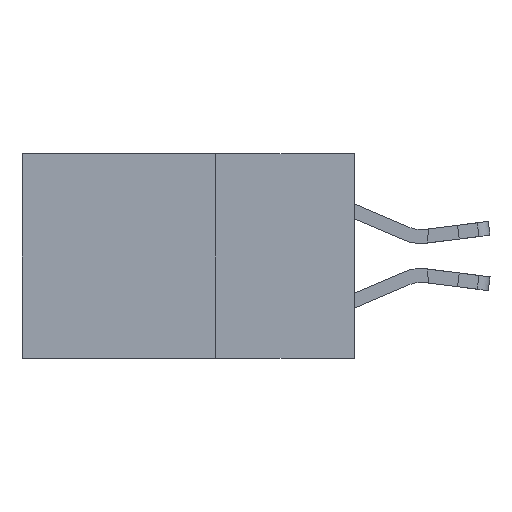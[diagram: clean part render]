
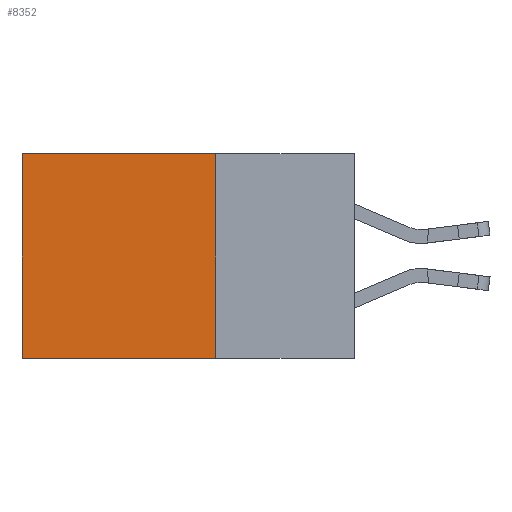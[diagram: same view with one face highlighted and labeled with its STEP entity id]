
A CAD part, left-side view. The second image highlights one B-rep face of the part: STEP entity #8352.
In plain terms, the highlighted planar face has unit normal (-1, 0, 0).
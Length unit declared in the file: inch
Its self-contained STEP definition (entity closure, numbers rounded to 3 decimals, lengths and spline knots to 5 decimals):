
#589 = ORIENTED_EDGE ( 'NONE', *, *, #4561, .T. ) ;
#752 = CARTESIAN_POINT ( 'NONE',  ( 0.2615, 0.25, -0.37 ) ) ;
#1234 = CARTESIAN_POINT ( 'NONE',  ( 0.2615, 0.25, 0. ) ) ;
#1508 = VERTEX_POINT ( 'NONE', #752 ) ;
#2051 = CARTESIAN_POINT ( 'NONE',  ( 0.2615, 0.25, -0.37 ) ) ;
#2135 = DIRECTION ( 'NONE',  ( 0., 1., 0. ) ) ;
#2489 = LINE ( 'NONE', #11276, #8915 ) ;
#3273 = FACE_OUTER_BOUND ( 'NONE', #4015, .T. ) ;
#3302 = VERTEX_POINT ( 'NONE', #12610 ) ;
#3388 = DIRECTION ( 'NONE',  ( 0., 1., 0. ) ) ;
#3505 = CARTESIAN_POINT ( 'NONE',  ( 0.2615, 0.25, 0. ) ) ;
#4015 = EDGE_LOOP ( 'NONE', ( #11165, #12645, #15702, #589 ) ) ;
#4561 = EDGE_CURVE ( 'NONE', #10073, #11899, #10612, .T. ) ;
#5086 = CARTESIAN_POINT ( 'NONE',  ( 0.2615, 0.25, -0.37 ) ) ;
#5188 = DIRECTION ( 'NONE',  ( 0., 0., -1. ) ) ;
#7683 = EDGE_CURVE ( 'NONE', #10073, #1508, #8929, .T. ) ;
#8352 = ADVANCED_FACE ( 'NONE', ( #3273 ), #13591, .F. ) ;
#8394 = AXIS2_PLACEMENT_3D ( 'NONE', #13585, #13384, #13372 ) ;
#8647 = EDGE_CURVE ( 'NONE', #11899, #3302, #2489, .T. ) ;
#8915 = VECTOR ( 'NONE', #11234, 39.37008 ) ;
#8929 = LINE ( 'NONE', #5086, #11982 ) ;
#9011 = VECTOR ( 'NONE', #2135, 39.37008 ) ;
#9355 = VECTOR ( 'NONE', #3388, 39.37008 ) ;
#10073 = VERTEX_POINT ( 'NONE', #1234 ) ;
#10277 = CARTESIAN_POINT ( 'NONE',  ( 0.2615, 0.6, 0. ) ) ;
#10612 = LINE ( 'NONE', #3505, #9355 ) ;
#11165 = ORIENTED_EDGE ( 'NONE', *, *, #8647, .T. ) ;
#11234 = DIRECTION ( 'NONE',  ( 0., 0., -1. ) ) ;
#11276 = CARTESIAN_POINT ( 'NONE',  ( 0.2615, 0.6, -0.37 ) ) ;
#11655 = EDGE_CURVE ( 'NONE', #1508, #3302, #12462, .T. ) ;
#11899 = VERTEX_POINT ( 'NONE', #10277 ) ;
#11982 = VECTOR ( 'NONE', #5188, 39.37008 ) ;
#12462 = LINE ( 'NONE', #2051, #9011 ) ;
#12610 = CARTESIAN_POINT ( 'NONE',  ( 0.2615, 0.6, -0.37 ) ) ;
#12645 = ORIENTED_EDGE ( 'NONE', *, *, #11655, .F. ) ;
#13372 = DIRECTION ( 'NONE',  ( 0., 0., -1. ) ) ;
#13384 = DIRECTION ( 'NONE',  ( 1., 0., 0. ) ) ;
#13585 = CARTESIAN_POINT ( 'NONE',  ( 0.2615, 0.25, -0.37 ) ) ;
#13591 = PLANE ( 'NONE',  #8394 ) ;
#15702 = ORIENTED_EDGE ( 'NONE', *, *, #7683, .F. ) ;
